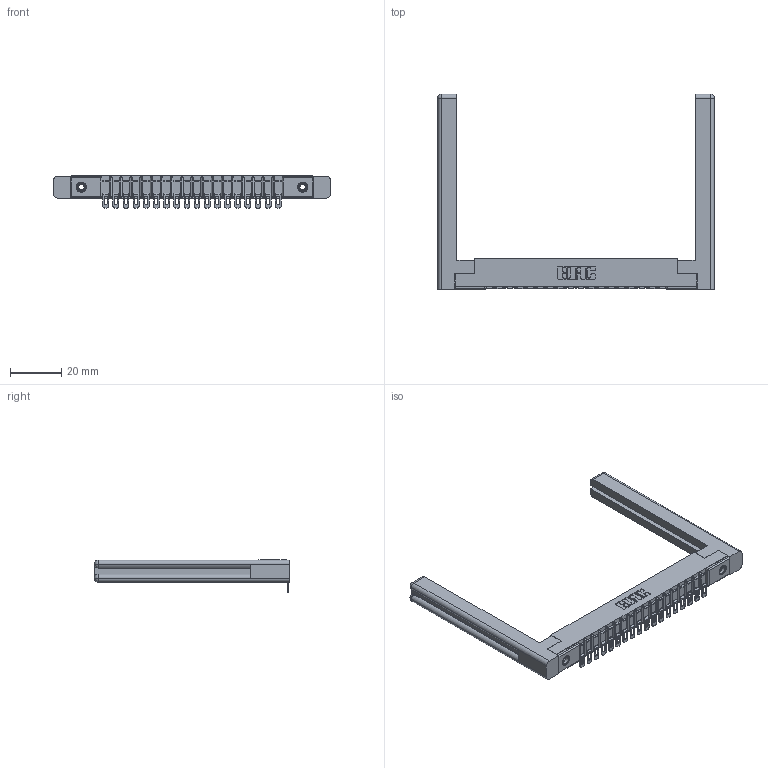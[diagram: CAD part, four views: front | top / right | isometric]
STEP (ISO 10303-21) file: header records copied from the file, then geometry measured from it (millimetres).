
FILE_DESCRIPTION (( 'STEP AP203' ), '1' );
FILE_NAME ('307-018-554-158.STEP', '2019-09-04T22:23:12', ( '' ), ( '' ), 'SwSTEP 2.0', 'SolidWorks 2016', '' );
FILE_SCHEMA (( 'CONFIG_CONTROL_DESIGN' ));
Length unit declared in the file: inch
Products named in the file (5): 307-220-058; 307-290-002_554; 345-250-001_345-250-001-102; 307-018-554-158; 307 Part_.156 Dia Mounting Holes
Assembly tree (23 placements, depth 2):
  307-018-554-158
    307 Part_.156 Dia Mounting Holes
    307-290-002_554  x18
    307-220-058  x2
    345-250-001_345-250-001-102  x2
Bounding box: 107.95 x 76.33 x 12.52 mm (x, y, z)
Volume: 14809.4 mm3; surface area: 17846.2 mm2
Topology: 23 solids, 23 shells, 1737 faces, 5231 edges, 3422 vertices
Faces by surface type: plane 982, cylinder 693, sphere 38, torus 12, cone 12
Entity records: 21988 total; most frequent: CARTESIAN_POINT 3713, ORIENTED_EDGE 3642, DIRECTION 3585, EDGE_CURVE 1821, VECTOR 1373, LINE 1373, VERTEX_POINT 1180, AXIS2_PLACEMENT_3D 1106
